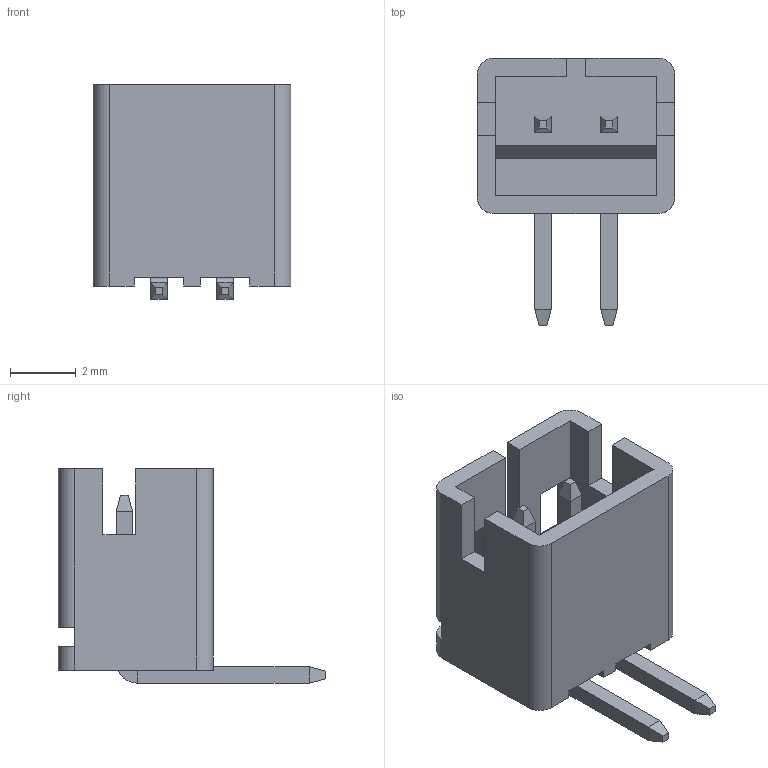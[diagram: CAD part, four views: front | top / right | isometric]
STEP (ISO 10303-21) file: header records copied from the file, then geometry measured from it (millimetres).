
FILE_DESCRIPTION (( 'STEP AP203' ), '1' );
FILE_NAME ('140-502-415-100.STEP', '2020-09-25T10:58:46', ( '' ), ( '' ), 'SwSTEP 2.0', 'SolidWorks 2020', '' );
FILE_SCHEMA (( 'CONFIG_CONTROL_DESIGN' ));
Length unit declared in the file: millimetre
Products named in the file (3): RA LI Contact_Str; 140-502-415-100; RA LI Housing_502
Assembly tree (3 placements, depth 2):
  140-502-415-100
    RA LI Housing_502
    RA LI Contact_Str  x2
Bounding box: 6 x 8.1 x 6.5 mm (x, y, z)
Volume: 82.9 mm3; surface area: 313.5 mm2
Topology: 3 solids, 3 shells, 100 faces, 252 edges, 156 vertices
Faces by surface type: plane 90, cylinder 10
Entity records: 2721 total; most frequent: CARTESIAN_POINT 424, ORIENTED_EDGE 416, DIRECTION 392, EDGE_CURVE 208, VECTOR 192, LINE 192, VERTEX_POINT 132, AXIS2_PLACEMENT_3D 100
